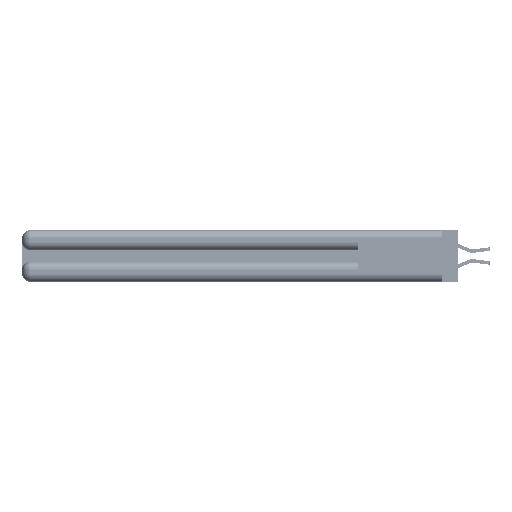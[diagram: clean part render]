
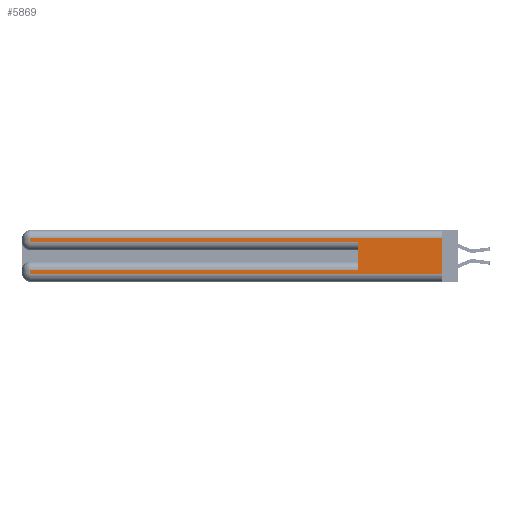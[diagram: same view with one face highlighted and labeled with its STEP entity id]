
A CAD part, left-side view. The second image highlights one B-rep face of the part: STEP entity #5869.
In plain terms, the highlighted planar face has unit normal (-1, 0, 0).
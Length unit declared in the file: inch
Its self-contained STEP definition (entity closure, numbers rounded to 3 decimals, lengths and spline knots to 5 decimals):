
#1205 = DIRECTION ( 'NONE',  ( 0., 0., -1. ) ) ;
#1801 = CARTESIAN_POINT ( 'NONE',  ( 0., 2.94, 0.37 ) ) ;
#2867 = EDGE_CURVE ( 'NONE', #6243, #39973, #8561, .T. ) ;
#3347 = LINE ( 'NONE', #1801, #14055 ) ;
#3382 = DIRECTION ( 'NONE',  ( 0., 0., -1. ) ) ;
#3538 = VERTEX_POINT ( 'NONE', #28295 ) ;
#3826 = LINE ( 'NONE', #9884, #40780 ) ;
#5570 = VECTOR ( 'NONE', #1205, 39.37008 ) ;
#5869 = ADVANCED_FACE ( 'NONE', ( #36909 ), #42337, .F. ) ;
#6243 = VERTEX_POINT ( 'NONE', #30655 ) ;
#6317 = VECTOR ( 'NONE', #3382, 39.37008 ) ;
#6439 = DIRECTION ( 'NONE',  ( 0., -1., 0. ) ) ;
#6793 = LINE ( 'NONE', #31425, #42599 ) ;
#8561 = LINE ( 'NONE', #46232, #6317 ) ;
#9073 = DIRECTION ( 'NONE',  ( 0., 0., -1. ) ) ;
#9376 = ORIENTED_EDGE ( 'NONE', *, *, #42299, .T. ) ;
#9486 = CARTESIAN_POINT ( 'NONE',  ( 0., 2.94, 0.085 ) ) ;
#9884 = CARTESIAN_POINT ( 'NONE',  ( 0., 0., 0.285 ) ) ;
#10465 = DIRECTION ( 'NONE',  ( 1., 0., 0. ) ) ;
#13805 = VERTEX_POINT ( 'NONE', #25914 ) ;
#13888 = EDGE_CURVE ( 'NONE', #13805, #41272, #24685, .T. ) ;
#14055 = VECTOR ( 'NONE', #9073, 39.37008 ) ;
#15659 = CARTESIAN_POINT ( 'NONE',  ( 0., 0., 0.06 ) ) ;
#17144 = VECTOR ( 'NONE', #21177, 39.37008 ) ;
#17564 = CARTESIAN_POINT ( 'NONE',  ( 0., 0., 0.085 ) ) ;
#17938 = DIRECTION ( 'NONE',  ( 0., -1., 0. ) ) ;
#17967 = ORIENTED_EDGE ( 'NONE', *, *, #23370, .T. ) ;
#18518 = CARTESIAN_POINT ( 'NONE',  ( 0., 0.6, 0.145 ) ) ;
#20278 = EDGE_CURVE ( 'NONE', #30704, #24141, #45623, .T. ) ;
#20765 = CARTESIAN_POINT ( 'NONE',  ( 0., 0.6, 0.085 ) ) ;
#21177 = DIRECTION ( 'NONE',  ( 0., 1., 0. ) ) ;
#23370 = EDGE_CURVE ( 'NONE', #24141, #39201, #3347, .T. ) ;
#23981 = ORIENTED_EDGE ( 'NONE', *, *, #20278, .T. ) ;
#24141 = VERTEX_POINT ( 'NONE', #9486 ) ;
#24331 = CARTESIAN_POINT ( 'NONE',  ( 0., 2.94, 0.285 ) ) ;
#24611 = AXIS2_PLACEMENT_3D ( 'NONE', #28354, #10465, #35515 ) ;
#24685 = LINE ( 'NONE', #33435, #5570 ) ;
#25914 = CARTESIAN_POINT ( 'NONE',  ( 0., 0., 0.31 ) ) ;
#26476 = LINE ( 'NONE', #18518, #27615 ) ;
#26800 = EDGE_CURVE ( 'NONE', #30704, #3538, #26476, .T. ) ;
#26858 = EDGE_LOOP ( 'NONE', ( #29773, #36395, #27833, #41037, #40769, #23981, #17967, #9376 ) ) ;
#27615 = VECTOR ( 'NONE', #32934, 39.37008 ) ;
#27661 = DIRECTION ( 'NONE',  ( 0., 1., 0. ) ) ;
#27833 = ORIENTED_EDGE ( 'NONE', *, *, #2867, .T. ) ;
#28295 = CARTESIAN_POINT ( 'NONE',  ( 0., 0.6, 0.285 ) ) ;
#28354 = CARTESIAN_POINT ( 'NONE',  ( 0., 0., 0.37 ) ) ;
#29773 = ORIENTED_EDGE ( 'NONE', *, *, #13888, .F. ) ;
#30655 = CARTESIAN_POINT ( 'NONE',  ( 0., 2.94, 0.31 ) ) ;
#30704 = VERTEX_POINT ( 'NONE', #20765 ) ;
#31425 = CARTESIAN_POINT ( 'NONE',  ( 0., 0., 0.31 ) ) ;
#32934 = DIRECTION ( 'NONE',  ( 0., 0., 1. ) ) ;
#33435 = CARTESIAN_POINT ( 'NONE',  ( 0., 0., 0.37 ) ) ;
#35515 = DIRECTION ( 'NONE',  ( 0., 0., -1. ) ) ;
#36103 = EDGE_CURVE ( 'NONE', #13805, #6243, #6793, .T. ) ;
#36395 = ORIENTED_EDGE ( 'NONE', *, *, #36103, .T. ) ;
#36575 = VECTOR ( 'NONE', #17938, 39.37008 ) ;
#36909 = FACE_OUTER_BOUND ( 'NONE', #26858, .T. ) ;
#38096 = EDGE_CURVE ( 'NONE', #39973, #3538, #3826, .T. ) ;
#39201 = VERTEX_POINT ( 'NONE', #44009 ) ;
#39973 = VERTEX_POINT ( 'NONE', #24331 ) ;
#40769 = ORIENTED_EDGE ( 'NONE', *, *, #26800, .F. ) ;
#40780 = VECTOR ( 'NONE', #6439, 39.37008 ) ;
#41037 = ORIENTED_EDGE ( 'NONE', *, *, #38096, .T. ) ;
#41272 = VERTEX_POINT ( 'NONE', #15659 ) ;
#42299 = EDGE_CURVE ( 'NONE', #39201, #41272, #44890, .T. ) ;
#42337 = PLANE ( 'NONE',  #24611 ) ;
#42599 = VECTOR ( 'NONE', #27661, 39.37008 ) ;
#42892 = CARTESIAN_POINT ( 'NONE',  ( 0., 0., 0.06 ) ) ;
#44009 = CARTESIAN_POINT ( 'NONE',  ( 0., 2.94, 0.06 ) ) ;
#44890 = LINE ( 'NONE', #42892, #36575 ) ;
#45623 = LINE ( 'NONE', #17564, #17144 ) ;
#46232 = CARTESIAN_POINT ( 'NONE',  ( 0., 2.94, 0.37 ) ) ;
